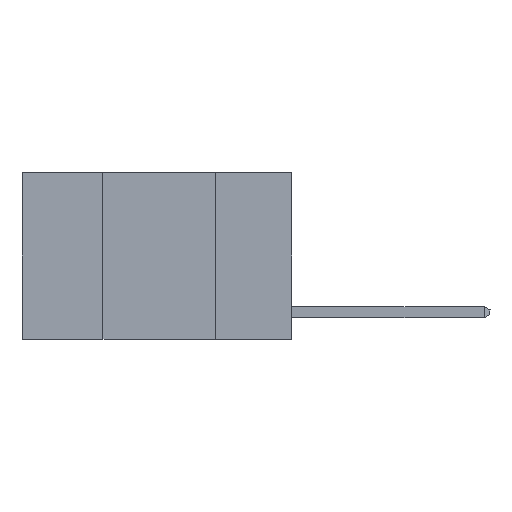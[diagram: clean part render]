
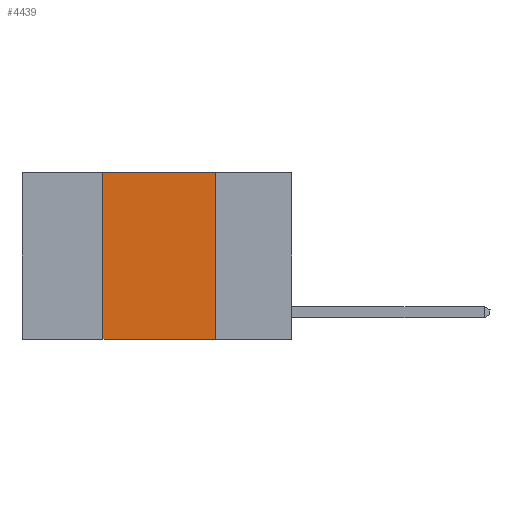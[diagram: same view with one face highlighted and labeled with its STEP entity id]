
A CAD part, left-side view. The second image highlights one B-rep face of the part: STEP entity #4439.
In plain terms, the highlighted planar face has unit normal (-1, 0, 0).
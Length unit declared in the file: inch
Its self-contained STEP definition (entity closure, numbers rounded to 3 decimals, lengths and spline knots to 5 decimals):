
#94 = VERTEX_POINT ( 'NONE', #9404 ) ;
#180 = VERTEX_POINT ( 'NONE', #11563 ) ;
#541 = CARTESIAN_POINT ( 'NONE',  ( 0., 0.17, 0. ) ) ;
#878 = LINE ( 'NONE', #541, #15589 ) ;
#1353 = PLANE ( 'NONE',  #11657 ) ;
#1496 = EDGE_CURVE ( 'NONE', #94, #5260, #878, .T. ) ;
#1515 = EDGE_CURVE ( 'NONE', #6588, #5260, #12275, .T. ) ;
#1867 = EDGE_CURVE ( 'NONE', #6588, #180, #2231, .T. ) ;
#2231 = LINE ( 'NONE', #10810, #6097 ) ;
#2914 = CARTESIAN_POINT ( 'NONE',  ( 0., 0.6, 0. ) ) ;
#3322 = FACE_OUTER_BOUND ( 'NONE', #3578, .T. ) ;
#3356 = ORIENTED_EDGE ( 'NONE', *, *, #1496, .F. ) ;
#3578 = EDGE_LOOP ( 'NONE', ( #3356, #10899, #14638, #18403 ) ) ;
#4367 = DIRECTION ( 'NONE',  ( 0., 0., -1. ) ) ;
#4439 = ADVANCED_FACE ( 'NONE', ( #3322 ), #1353, .F. ) ;
#5260 = VERTEX_POINT ( 'NONE', #13411 ) ;
#6097 = VECTOR ( 'NONE', #10568, 39.37008 ) ;
#6274 = DIRECTION ( 'NONE',  ( 0., -1., 0. ) ) ;
#6588 = VERTEX_POINT ( 'NONE', #17789 ) ;
#9404 = CARTESIAN_POINT ( 'NONE',  ( 0., 0.17, 0. ) ) ;
#10568 = DIRECTION ( 'NONE',  ( 0., 0., 1. ) ) ;
#10810 = CARTESIAN_POINT ( 'NONE',  ( 0., 0.42, 0. ) ) ;
#10899 = ORIENTED_EDGE ( 'NONE', *, *, #11176, .F. ) ;
#11176 = EDGE_CURVE ( 'NONE', #180, #94, #17825, .T. ) ;
#11563 = CARTESIAN_POINT ( 'NONE',  ( 0., 0.42, 0. ) ) ;
#11657 = AXIS2_PLACEMENT_3D ( 'NONE', #2914, #12835, #4367 ) ;
#11828 = VECTOR ( 'NONE', #16052, 39.37008 ) ;
#12275 = LINE ( 'NONE', #16047, #11828 ) ;
#12835 = DIRECTION ( 'NONE',  ( 1., 0., 0. ) ) ;
#13295 = CARTESIAN_POINT ( 'NONE',  ( 0., 0.6, 0. ) ) ;
#13411 = CARTESIAN_POINT ( 'NONE',  ( 0., 0.17, -0.37 ) ) ;
#13653 = VECTOR ( 'NONE', #6274, 39.37008 ) ;
#14638 = ORIENTED_EDGE ( 'NONE', *, *, #1867, .F. ) ;
#15589 = VECTOR ( 'NONE', #17765, 39.37008 ) ;
#16047 = CARTESIAN_POINT ( 'NONE',  ( 0., 0.6, -0.37 ) ) ;
#16052 = DIRECTION ( 'NONE',  ( 0., -1., 0. ) ) ;
#17765 = DIRECTION ( 'NONE',  ( 0., 0., -1. ) ) ;
#17789 = CARTESIAN_POINT ( 'NONE',  ( 0., 0.42, -0.37 ) ) ;
#17825 = LINE ( 'NONE', #13295, #13653 ) ;
#18403 = ORIENTED_EDGE ( 'NONE', *, *, #1515, .T. ) ;
